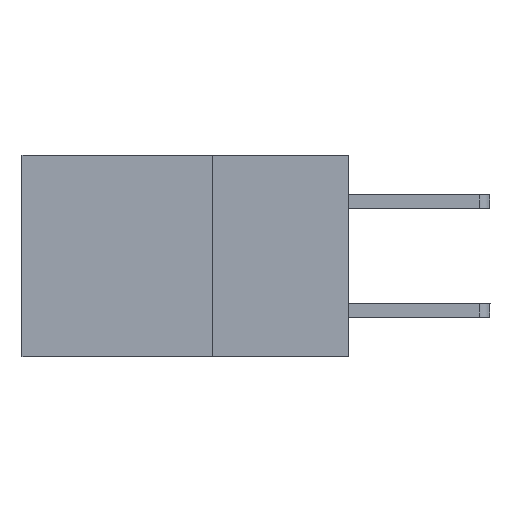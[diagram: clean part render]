
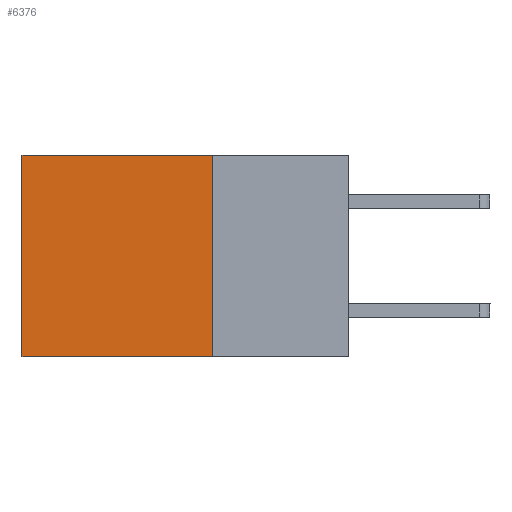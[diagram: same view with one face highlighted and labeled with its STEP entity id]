
A CAD part, left-side view. The second image highlights one B-rep face of the part: STEP entity #6376.
In plain terms, the highlighted planar face has unit normal (-1, 0, 0).
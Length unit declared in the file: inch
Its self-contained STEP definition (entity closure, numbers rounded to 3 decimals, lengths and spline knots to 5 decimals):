
#135 = CARTESIAN_POINT ( 'NONE',  ( 0.298, 0.25, 0. ) ) ;
#700 = CARTESIAN_POINT ( 'NONE',  ( 0.298, 0.25, 0. ) ) ;
#843 = DIRECTION ( 'NONE',  ( 0., 0., -1. ) ) ;
#1013 = VECTOR ( 'NONE', #3954, 39.37008 ) ;
#1474 = VERTEX_POINT ( 'NONE', #10311 ) ;
#1543 = VECTOR ( 'NONE', #4347, 39.37008 ) ;
#2004 = DIRECTION ( 'NONE',  ( 0., 0., -1. ) ) ;
#2492 = ORIENTED_EDGE ( 'NONE', *, *, #9672, .F. ) ;
#2771 = VECTOR ( 'NONE', #843, 39.37008 ) ;
#2832 = LINE ( 'NONE', #700, #6403 ) ;
#3314 = LINE ( 'NONE', #5124, #2771 ) ;
#3834 = ORIENTED_EDGE ( 'NONE', *, *, #9117, .T. ) ;
#3874 = LINE ( 'NONE', #9471, #1543 ) ;
#3954 = DIRECTION ( 'NONE',  ( 0., 1., 0. ) ) ;
#4347 = DIRECTION ( 'NONE',  ( 0., 1., 0. ) ) ;
#5124 = CARTESIAN_POINT ( 'NONE',  ( 0.298, 0.6, 0. ) ) ;
#5260 = PLANE ( 'NONE',  #6382 ) ;
#6376 = ADVANCED_FACE ( 'NONE', ( #6492 ), #5260, .F. ) ;
#6382 = AXIS2_PLACEMENT_3D ( 'NONE', #135, #7843, #2004 ) ;
#6403 = VECTOR ( 'NONE', #6872, 39.37008 ) ;
#6492 = FACE_OUTER_BOUND ( 'NONE', #6842, .T. ) ;
#6584 = VERTEX_POINT ( 'NONE', #8060 ) ;
#6842 = EDGE_LOOP ( 'NONE', ( #6937, #2492, #9802, #3834 ) ) ;
#6872 = DIRECTION ( 'NONE',  ( 0., 0., -1. ) ) ;
#6937 = ORIENTED_EDGE ( 'NONE', *, *, #8703, .T. ) ;
#7626 = VERTEX_POINT ( 'NONE', #7831 ) ;
#7748 = VERTEX_POINT ( 'NONE', #9045 ) ;
#7831 = CARTESIAN_POINT ( 'NONE',  ( 0.298, 0.6, 0. ) ) ;
#7843 = DIRECTION ( 'NONE',  ( 1., 0., 0. ) ) ;
#8060 = CARTESIAN_POINT ( 'NONE',  ( 0.298, 0.25, -0.37 ) ) ;
#8210 = CARTESIAN_POINT ( 'NONE',  ( 0.298, 0.25, 0. ) ) ;
#8703 = EDGE_CURVE ( 'NONE', #7626, #7748, #3314, .T. ) ;
#9045 = CARTESIAN_POINT ( 'NONE',  ( 0.298, 0.6, -0.37 ) ) ;
#9117 = EDGE_CURVE ( 'NONE', #1474, #7626, #9566, .T. ) ;
#9471 = CARTESIAN_POINT ( 'NONE',  ( 0.298, 0.25, -0.37 ) ) ;
#9566 = LINE ( 'NONE', #8210, #1013 ) ;
#9672 = EDGE_CURVE ( 'NONE', #6584, #7748, #3874, .T. ) ;
#9802 = ORIENTED_EDGE ( 'NONE', *, *, #10719, .F. ) ;
#10311 = CARTESIAN_POINT ( 'NONE',  ( 0.298, 0.25, 0. ) ) ;
#10719 = EDGE_CURVE ( 'NONE', #1474, #6584, #2832, .T. ) ;
